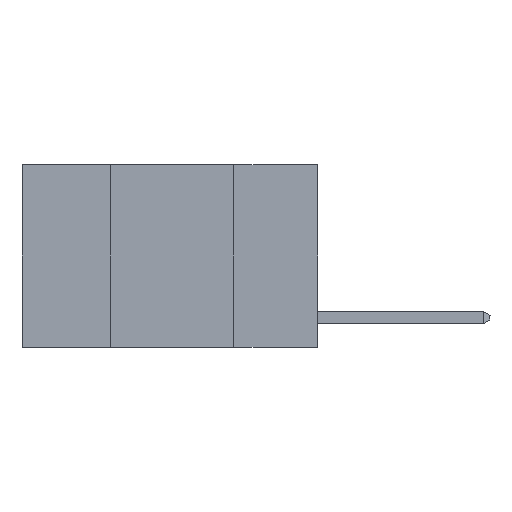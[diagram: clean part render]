
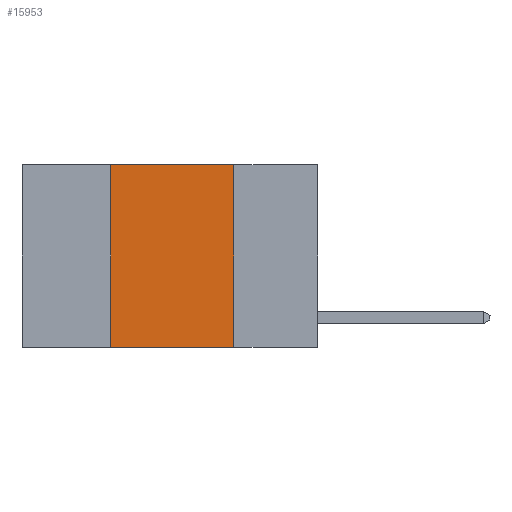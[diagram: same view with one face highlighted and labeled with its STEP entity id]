
A CAD part, left-side view. The second image highlights one B-rep face of the part: STEP entity #15953.
In plain terms, the highlighted planar face has unit normal (-1, 0, 0).
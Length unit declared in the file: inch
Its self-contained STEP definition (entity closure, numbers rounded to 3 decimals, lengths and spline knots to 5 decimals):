
#305 = EDGE_CURVE ( 'NONE', #6071, #4558, #6091, .T. ) ;
#409 = CARTESIAN_POINT ( 'NONE',  ( 0., 0.42, 0. ) ) ;
#462 = CARTESIAN_POINT ( 'NONE',  ( 0., 0.6, 0. ) ) ;
#813 = EDGE_CURVE ( 'NONE', #8477, #12778, #6534, .T. ) ;
#1178 = VECTOR ( 'NONE', #6335, 39.37008 ) ;
#3567 = CARTESIAN_POINT ( 'NONE',  ( 0., 0.42, -0.37 ) ) ;
#3676 = DIRECTION ( 'NONE',  ( 0., 0., -1. ) ) ;
#4128 = ORIENTED_EDGE ( 'NONE', *, *, #813, .F. ) ;
#4558 = VERTEX_POINT ( 'NONE', #5557 ) ;
#4751 = EDGE_CURVE ( 'NONE', #12778, #6071, #12174, .T. ) ;
#5048 = FACE_OUTER_BOUND ( 'NONE', #9272, .T. ) ;
#5377 = DIRECTION ( 'NONE',  ( 1., 0., 0. ) ) ;
#5557 = CARTESIAN_POINT ( 'NONE',  ( 0., 0.17, -0.37 ) ) ;
#6071 = VERTEX_POINT ( 'NONE', #8608 ) ;
#6091 = LINE ( 'NONE', #9899, #14453 ) ;
#6099 = LINE ( 'NONE', #9909, #1178 ) ;
#6335 = DIRECTION ( 'NONE',  ( 0., -1., 0. ) ) ;
#6534 = LINE ( 'NONE', #409, #8375 ) ;
#6589 = ORIENTED_EDGE ( 'NONE', *, *, #305, .F. ) ;
#8375 = VECTOR ( 'NONE', #10278, 39.37008 ) ;
#8477 = VERTEX_POINT ( 'NONE', #3567 ) ;
#8608 = CARTESIAN_POINT ( 'NONE',  ( 0., 0.17, 0. ) ) ;
#8884 = EDGE_CURVE ( 'NONE', #8477, #4558, #6099, .T. ) ;
#9061 = VECTOR ( 'NONE', #9832, 39.37008 ) ;
#9272 = EDGE_LOOP ( 'NONE', ( #6589, #13170, #4128, #11152 ) ) ;
#9832 = DIRECTION ( 'NONE',  ( 0., -1., 0. ) ) ;
#9899 = CARTESIAN_POINT ( 'NONE',  ( 0., 0.17, 0. ) ) ;
#9909 = CARTESIAN_POINT ( 'NONE',  ( 0., 0.6, -0.37 ) ) ;
#10278 = DIRECTION ( 'NONE',  ( 0., 0., 1. ) ) ;
#10299 = AXIS2_PLACEMENT_3D ( 'NONE', #462, #5377, #13778 ) ;
#11152 = ORIENTED_EDGE ( 'NONE', *, *, #8884, .T. ) ;
#11533 = PLANE ( 'NONE',  #10299 ) ;
#12174 = LINE ( 'NONE', #13297, #9061 ) ;
#12778 = VERTEX_POINT ( 'NONE', #13380 ) ;
#13170 = ORIENTED_EDGE ( 'NONE', *, *, #4751, .F. ) ;
#13297 = CARTESIAN_POINT ( 'NONE',  ( 0., 0.6, 0. ) ) ;
#13380 = CARTESIAN_POINT ( 'NONE',  ( 0., 0.42, 0. ) ) ;
#13778 = DIRECTION ( 'NONE',  ( 0., 0., -1. ) ) ;
#14453 = VECTOR ( 'NONE', #3676, 39.37008 ) ;
#15953 = ADVANCED_FACE ( 'NONE', ( #5048 ), #11533, .F. ) ;
